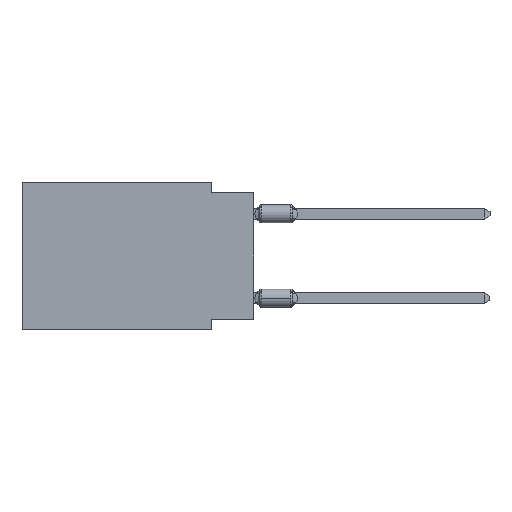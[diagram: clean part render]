
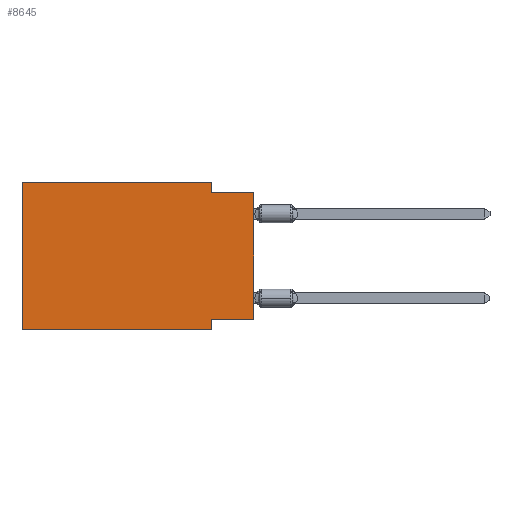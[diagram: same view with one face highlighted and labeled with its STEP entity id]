
A CAD part, left-side view. The second image highlights one B-rep face of the part: STEP entity #8645.
In plain terms, the highlighted planar face has unit normal (-1, 0, 0).
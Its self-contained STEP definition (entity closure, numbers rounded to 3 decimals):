
#212 = CARTESIAN_POINT ( 'NONE',  ( 0., 13.97, -8.89 ) ) ;
#432 = DIRECTION ( 'NONE',  ( 0., 0., -1. ) ) ;
#982 = VERTEX_POINT ( 'NONE', #12575 ) ;
#1028 = LINE ( 'NONE', #11547, #11023 ) ;
#1195 = DIRECTION ( 'NONE',  ( 0., -1., 0. ) ) ;
#1307 = EDGE_CURVE ( 'NONE', #7655, #7501, #11110, .T. ) ;
#1432 = ORIENTED_EDGE ( 'NONE', *, *, #1307, .F. ) ;
#1578 = EDGE_CURVE ( 'NONE', #2376, #3905, #7847, .T. ) ;
#1614 = CARTESIAN_POINT ( 'NONE',  ( 0., 2.54, -8.89 ) ) ;
#1966 = DIRECTION ( 'NONE',  ( 0., 0., 1. ) ) ;
#2301 = EDGE_CURVE ( 'NONE', #11842, #2376, #1028, .T. ) ;
#2376 = VERTEX_POINT ( 'NONE', #10859 ) ;
#2650 = EDGE_CURVE ( 'NONE', #7501, #6572, #4794, .T. ) ;
#2667 = PLANE ( 'NONE',  #8923 ) ;
#2740 = CARTESIAN_POINT ( 'NONE',  ( 0., 13.97, 0. ) ) ;
#3099 = EDGE_CURVE ( 'NONE', #4263, #3905, #6477, .T. ) ;
#3905 = VERTEX_POINT ( 'NONE', #13522 ) ;
#4263 = VERTEX_POINT ( 'NONE', #11374 ) ;
#4690 = VECTOR ( 'NONE', #5544, 1000. ) ;
#4744 = EDGE_LOOP ( 'NONE', ( #10689, #7265, #1432, #11714, #8384, #11800, #5667, #7167 ) ) ;
#4794 = LINE ( 'NONE', #10166, #11471 ) ;
#5302 = VECTOR ( 'NONE', #5880, 1000. ) ;
#5544 = DIRECTION ( 'NONE',  ( 0., 0., 1. ) ) ;
#5575 = CARTESIAN_POINT ( 'NONE',  ( 0., 0., -8.255 ) ) ;
#5667 = ORIENTED_EDGE ( 'NONE', *, *, #1578, .F. ) ;
#5880 = DIRECTION ( 'NONE',  ( 0., 0., -1. ) ) ;
#5885 = CARTESIAN_POINT ( 'NONE',  ( 0., 13.97, 0. ) ) ;
#5984 = EDGE_CURVE ( 'NONE', #4263, #982, #6637, .T. ) ;
#6114 = DIRECTION ( 'NONE',  ( 0., 1., 0. ) ) ;
#6477 = LINE ( 'NONE', #212, #12784 ) ;
#6545 = VECTOR ( 'NONE', #9325, 1000. ) ;
#6572 = VERTEX_POINT ( 'NONE', #8892 ) ;
#6637 = LINE ( 'NONE', #10766, #4690 ) ;
#6992 = DIRECTION ( 'NONE',  ( 0., 0., -1. ) ) ;
#7167 = ORIENTED_EDGE ( 'NONE', *, *, #2301, .F. ) ;
#7265 = ORIENTED_EDGE ( 'NONE', *, *, #2650, .F. ) ;
#7501 = VERTEX_POINT ( 'NONE', #13150 ) ;
#7655 = VERTEX_POINT ( 'NONE', #7790 ) ;
#7790 = CARTESIAN_POINT ( 'NONE',  ( 0., 2.54, 0. ) ) ;
#7847 = LINE ( 'NONE', #1614, #8819 ) ;
#8025 = DIRECTION ( 'NONE',  ( 1., 0., 0. ) ) ;
#8384 = ORIENTED_EDGE ( 'NONE', *, *, #5984, .F. ) ;
#8645 = ADVANCED_FACE ( 'NONE', ( #11127 ), #2667, .F. ) ;
#8819 = VECTOR ( 'NONE', #432, 1000. ) ;
#8892 = CARTESIAN_POINT ( 'NONE',  ( 0., 0., -0.635 ) ) ;
#8923 = AXIS2_PLACEMENT_3D ( 'NONE', #2740, #8025, #6992 ) ;
#9325 = DIRECTION ( 'NONE',  ( 0., -1., 0. ) ) ;
#9627 = EDGE_CURVE ( 'NONE', #982, #7655, #11310, .T. ) ;
#9654 = EDGE_CURVE ( 'NONE', #11842, #6572, #13363, .T. ) ;
#10166 = CARTESIAN_POINT ( 'NONE',  ( 0., 0., -0.635 ) ) ;
#10689 = ORIENTED_EDGE ( 'NONE', *, *, #9654, .T. ) ;
#10766 = CARTESIAN_POINT ( 'NONE',  ( 0., 13.97, 0. ) ) ;
#10859 = CARTESIAN_POINT ( 'NONE',  ( 0., 2.54, -8.255 ) ) ;
#11023 = VECTOR ( 'NONE', #6114, 1000. ) ;
#11110 = LINE ( 'NONE', #12336, #5302 ) ;
#11127 = FACE_OUTER_BOUND ( 'NONE', #4744, .T. ) ;
#11245 = CARTESIAN_POINT ( 'NONE',  ( 0., 0., 0. ) ) ;
#11310 = LINE ( 'NONE', #5885, #6545 ) ;
#11374 = CARTESIAN_POINT ( 'NONE',  ( 0., 13.97, -8.89 ) ) ;
#11471 = VECTOR ( 'NONE', #12080, 1000. ) ;
#11547 = CARTESIAN_POINT ( 'NONE',  ( 0., 0., -8.255 ) ) ;
#11714 = ORIENTED_EDGE ( 'NONE', *, *, #9627, .F. ) ;
#11800 = ORIENTED_EDGE ( 'NONE', *, *, #3099, .T. ) ;
#11842 = VERTEX_POINT ( 'NONE', #5575 ) ;
#12080 = DIRECTION ( 'NONE',  ( 0., -1., 0. ) ) ;
#12336 = CARTESIAN_POINT ( 'NONE',  ( 0., 2.54, 0. ) ) ;
#12481 = VECTOR ( 'NONE', #1966, 1000. ) ;
#12575 = CARTESIAN_POINT ( 'NONE',  ( 0., 13.97, 0. ) ) ;
#12784 = VECTOR ( 'NONE', #1195, 1000. ) ;
#13150 = CARTESIAN_POINT ( 'NONE',  ( 0., 2.54, -0.635 ) ) ;
#13363 = LINE ( 'NONE', #11245, #12481 ) ;
#13522 = CARTESIAN_POINT ( 'NONE',  ( 0., 2.54, -8.89 ) ) ;
